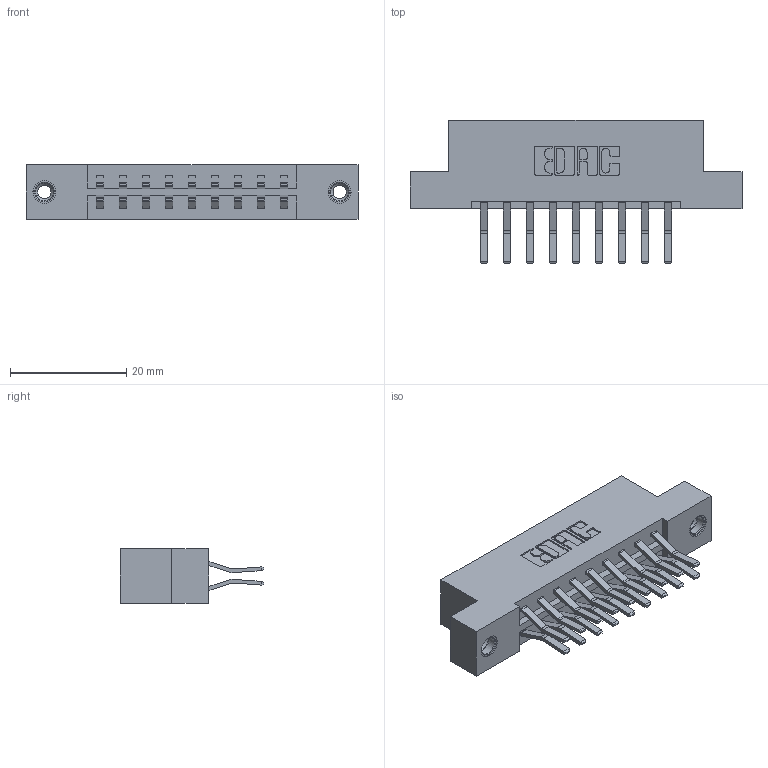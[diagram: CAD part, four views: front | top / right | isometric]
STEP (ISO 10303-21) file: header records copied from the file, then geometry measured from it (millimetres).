
FILE_DESCRIPTION (( 'STEP AP203' ), '1' );
FILE_NAME ('333-018-560-208.STEP', '2019-08-09T14:30:20', ( '' ), ( '' ), 'SwSTEP 2.0', 'SolidWorks 2016', '' );
FILE_SCHEMA (( 'CONFIG_CONTROL_DESIGN' ));
Length unit declared in the file: inch
Products named in the file (4): 333-018-560-208; 333 Part_Flush - .156 Dia - TI; 345-292-001_560 Tail; 345-250-001_345-250-003-102
Assembly tree (21 placements, depth 2):
  333-018-560-208
    333 Part_Flush - .156 Dia - TI
    345-292-001_560 Tail  x18
    345-250-001_345-250-003-102  x2
Bounding box: 57.2 x 24.78 x 9.4 mm (x, y, z)
Volume: 5642.7 mm3; surface area: 6674.8 mm2
Topology: 21 solids, 21 shells, 1146 faces, 3345 edges, 2198 vertices
Faces by surface type: plane 750, cylinder 380, cone 12, torus 4
Entity records: 11332 total; most frequent: CARTESIAN_POINT 1901, ORIENTED_EDGE 1830, DIRECTION 1717, EDGE_CURVE 915, LINE 763, VECTOR 763, VERTEX_POINT 604, AXIS2_PLACEMENT_3D 477
